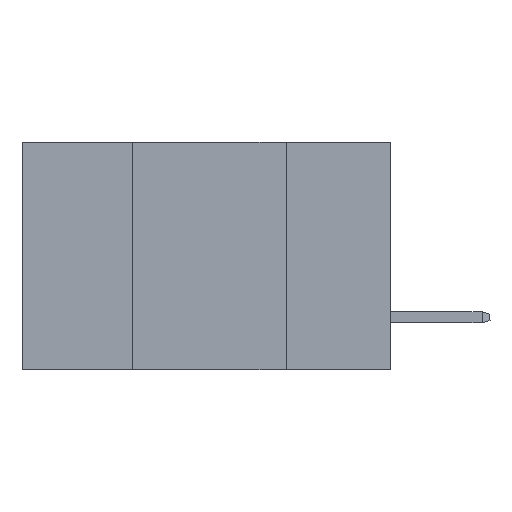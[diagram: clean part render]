
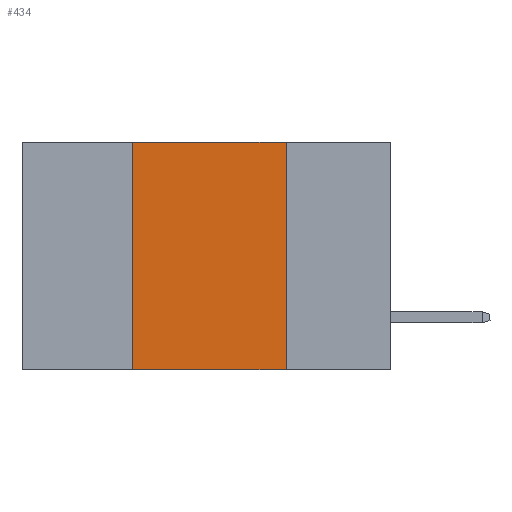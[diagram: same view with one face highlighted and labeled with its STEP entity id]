
A CAD part, left-side view. The second image highlights one B-rep face of the part: STEP entity #434.
In plain terms, the highlighted planar face has unit normal (-1, 0, 0).
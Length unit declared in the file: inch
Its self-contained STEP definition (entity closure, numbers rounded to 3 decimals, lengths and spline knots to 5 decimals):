
#362 = AXIS2_PLACEMENT_3D ( 'NONE', #8199, #8366, #5255 ) ;
#434 = ADVANCED_FACE ( 'NONE', ( #2130 ), #8683, .F. ) ;
#476 = CARTESIAN_POINT ( 'NONE',  ( 0., 0.6, 0. ) ) ;
#508 = DIRECTION ( 'NONE',  ( 0., -1., 0. ) ) ;
#648 = DIRECTION ( 'NONE',  ( 0., -1., 0. ) ) ;
#1102 = VECTOR ( 'NONE', #508, 39.37008 ) ;
#1231 = VECTOR ( 'NONE', #8787, 39.37008 ) ;
#1618 = LINE ( 'NONE', #2879, #7153 ) ;
#1751 = VERTEX_POINT ( 'NONE', #5906 ) ;
#2130 = FACE_OUTER_BOUND ( 'NONE', #4276, .T. ) ;
#2719 = EDGE_CURVE ( 'NONE', #7361, #7341, #3076, .T. ) ;
#2879 = CARTESIAN_POINT ( 'NONE',  ( 0., 0.42, 0. ) ) ;
#2943 = VERTEX_POINT ( 'NONE', #3697 ) ;
#3076 = LINE ( 'NONE', #7399, #1231 ) ;
#3697 = CARTESIAN_POINT ( 'NONE',  ( 0., 0.42, -0.37 ) ) ;
#4005 = CARTESIAN_POINT ( 'NONE',  ( 0., 0.17, -0.37 ) ) ;
#4276 = EDGE_LOOP ( 'NONE', ( #4655, #5258, #6237, #5091 ) ) ;
#4655 = ORIENTED_EDGE ( 'NONE', *, *, #2719, .F. ) ;
#4879 = DIRECTION ( 'NONE',  ( 0., 0., 1. ) ) ;
#5091 = ORIENTED_EDGE ( 'NONE', *, *, #5467, .T. ) ;
#5255 = DIRECTION ( 'NONE',  ( 0., 0., -1. ) ) ;
#5258 = ORIENTED_EDGE ( 'NONE', *, *, #8104, .F. ) ;
#5467 = EDGE_CURVE ( 'NONE', #2943, #7341, #6176, .T. ) ;
#5648 = EDGE_CURVE ( 'NONE', #2943, #1751, #1618, .T. ) ;
#5906 = CARTESIAN_POINT ( 'NONE',  ( 0., 0.42, 0. ) ) ;
#6176 = LINE ( 'NONE', #6852, #7689 ) ;
#6237 = ORIENTED_EDGE ( 'NONE', *, *, #5648, .F. ) ;
#6732 = LINE ( 'NONE', #476, #1102 ) ;
#6852 = CARTESIAN_POINT ( 'NONE',  ( 0., 0.6, -0.37 ) ) ;
#7153 = VECTOR ( 'NONE', #4879, 39.37008 ) ;
#7341 = VERTEX_POINT ( 'NONE', #4005 ) ;
#7361 = VERTEX_POINT ( 'NONE', #8120 ) ;
#7399 = CARTESIAN_POINT ( 'NONE',  ( 0., 0.17, 0. ) ) ;
#7689 = VECTOR ( 'NONE', #648, 39.37008 ) ;
#8104 = EDGE_CURVE ( 'NONE', #1751, #7361, #6732, .T. ) ;
#8120 = CARTESIAN_POINT ( 'NONE',  ( 0., 0.17, 0. ) ) ;
#8199 = CARTESIAN_POINT ( 'NONE',  ( 0., 0.6, 0. ) ) ;
#8366 = DIRECTION ( 'NONE',  ( 1., 0., 0. ) ) ;
#8683 = PLANE ( 'NONE',  #362 ) ;
#8787 = DIRECTION ( 'NONE',  ( 0., 0., -1. ) ) ;
